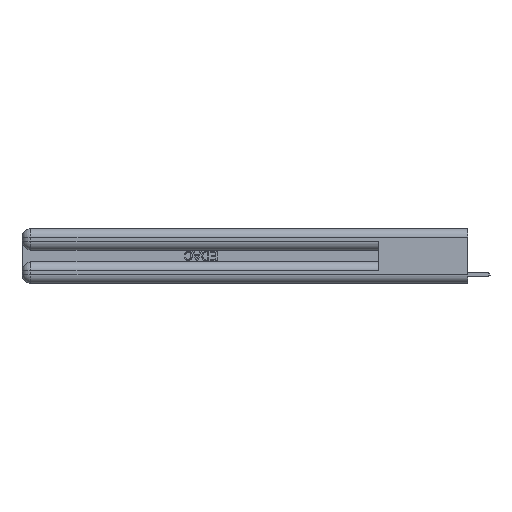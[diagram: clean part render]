
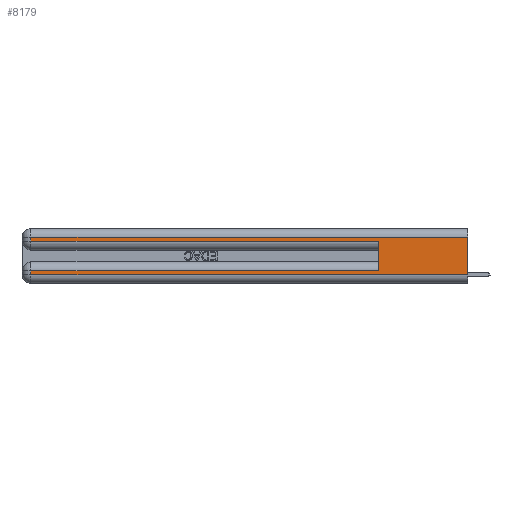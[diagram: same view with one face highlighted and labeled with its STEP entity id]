
A CAD part, left-side view. The second image highlights one B-rep face of the part: STEP entity #8179.
In plain terms, the highlighted planar face has unit normal (-1, 0, 0).
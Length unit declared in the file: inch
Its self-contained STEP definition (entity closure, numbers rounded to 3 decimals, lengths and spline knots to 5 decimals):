
#198 = CARTESIAN_POINT ( 'NONE',  ( 0., 0., 0.06 ) ) ;
#543 = CARTESIAN_POINT ( 'NONE',  ( 0., 2.94, 0.37 ) ) ;
#770 = CARTESIAN_POINT ( 'NONE',  ( 0., 0., 0.31 ) ) ;
#833 = VERTEX_POINT ( 'NONE', #26315 ) ;
#1070 = ORIENTED_EDGE ( 'NONE', *, *, #5201, .T. ) ;
#1204 = VECTOR ( 'NONE', #26337, 39.37008 ) ;
#1391 = VERTEX_POINT ( 'NONE', #16134 ) ;
#1666 = ORIENTED_EDGE ( 'NONE', *, *, #19985, .T. ) ;
#2874 = ORIENTED_EDGE ( 'NONE', *, *, #17030, .T. ) ;
#2978 = AXIS2_PLACEMENT_3D ( 'NONE', #25072, #17737, #20302 ) ;
#3149 = CARTESIAN_POINT ( 'NONE',  ( 0., 2.94, 0.31 ) ) ;
#3620 = PLANE ( 'NONE',  #2978 ) ;
#3633 = LINE ( 'NONE', #27394, #27458 ) ;
#4206 = ORIENTED_EDGE ( 'NONE', *, *, #17694, .F. ) ;
#4421 = VECTOR ( 'NONE', #28871, 39.37008 ) ;
#5201 = EDGE_CURVE ( 'NONE', #1391, #10972, #11929, .T. ) ;
#6618 = CARTESIAN_POINT ( 'NONE',  ( 0., 0., 0.285 ) ) ;
#6822 = VECTOR ( 'NONE', #21873, 39.37008 ) ;
#6922 = VECTOR ( 'NONE', #17334, 39.37008 ) ;
#7371 = CARTESIAN_POINT ( 'NONE',  ( 0., 2.94, 0.06 ) ) ;
#7586 = VERTEX_POINT ( 'NONE', #7646 ) ;
#7646 = CARTESIAN_POINT ( 'NONE',  ( 0., 0.6, 0.285 ) ) ;
#8179 = ADVANCED_FACE ( 'NONE', ( #18032 ), #3620, .F. ) ;
#8916 = LINE ( 'NONE', #24292, #22988 ) ;
#9814 = LINE ( 'NONE', #28670, #6922 ) ;
#9959 = EDGE_CURVE ( 'NONE', #13975, #1391, #9814, .T. ) ;
#10230 = LINE ( 'NONE', #770, #1204 ) ;
#10925 = LINE ( 'NONE', #6618, #19636 ) ;
#10972 = VERTEX_POINT ( 'NONE', #7371 ) ;
#11510 = CARTESIAN_POINT ( 'NONE',  ( 0., 2.94, 0.285 ) ) ;
#11929 = LINE ( 'NONE', #21104, #16793 ) ;
#12183 = VERTEX_POINT ( 'NONE', #18018 ) ;
#13900 = CARTESIAN_POINT ( 'NONE',  ( 0., 0.6, 0.085 ) ) ;
#13975 = VERTEX_POINT ( 'NONE', #13900 ) ;
#14807 = EDGE_CURVE ( 'NONE', #10972, #833, #29083, .T. ) ;
#15764 = ORIENTED_EDGE ( 'NONE', *, *, #18170, .F. ) ;
#15989 = DIRECTION ( 'NONE',  ( 0., 0., 1. ) ) ;
#16134 = CARTESIAN_POINT ( 'NONE',  ( 0., 2.94, 0.085 ) ) ;
#16192 = ORIENTED_EDGE ( 'NONE', *, *, #14807, .T. ) ;
#16793 = VECTOR ( 'NONE', #17137, 39.37008 ) ;
#17030 = EDGE_CURVE ( 'NONE', #24422, #19929, #19507, .T. ) ;
#17137 = DIRECTION ( 'NONE',  ( 0., 0., -1. ) ) ;
#17334 = DIRECTION ( 'NONE',  ( 0., 1., 0. ) ) ;
#17694 = EDGE_CURVE ( 'NONE', #12183, #833, #3633, .T. ) ;
#17737 = DIRECTION ( 'NONE',  ( 1., 0., 0. ) ) ;
#18018 = CARTESIAN_POINT ( 'NONE',  ( 0., 0., 0.31 ) ) ;
#18032 = FACE_OUTER_BOUND ( 'NONE', #22688, .T. ) ;
#18044 = DIRECTION ( 'NONE',  ( 0., 0., -1. ) ) ;
#18170 = EDGE_CURVE ( 'NONE', #13975, #7586, #8916, .T. ) ;
#19507 = LINE ( 'NONE', #543, #4421 ) ;
#19636 = VECTOR ( 'NONE', #30207, 39.37008 ) ;
#19929 = VERTEX_POINT ( 'NONE', #11510 ) ;
#19985 = EDGE_CURVE ( 'NONE', #19929, #7586, #10925, .T. ) ;
#20302 = DIRECTION ( 'NONE',  ( 0., 0., -1. ) ) ;
#21104 = CARTESIAN_POINT ( 'NONE',  ( 0., 2.94, 0.37 ) ) ;
#21404 = ORIENTED_EDGE ( 'NONE', *, *, #9959, .T. ) ;
#21873 = DIRECTION ( 'NONE',  ( 0., -1., 0. ) ) ;
#22688 = EDGE_LOOP ( 'NONE', ( #4206, #26595, #2874, #1666, #15764, #21404, #1070, #16192 ) ) ;
#22988 = VECTOR ( 'NONE', #15989, 39.37008 ) ;
#24292 = CARTESIAN_POINT ( 'NONE',  ( 0., 0.6, 0.145 ) ) ;
#24422 = VERTEX_POINT ( 'NONE', #3149 ) ;
#25072 = CARTESIAN_POINT ( 'NONE',  ( 0., 0., 0.37 ) ) ;
#26315 = CARTESIAN_POINT ( 'NONE',  ( 0., 0., 0.06 ) ) ;
#26337 = DIRECTION ( 'NONE',  ( 0., 1., 0. ) ) ;
#26595 = ORIENTED_EDGE ( 'NONE', *, *, #27722, .T. ) ;
#27394 = CARTESIAN_POINT ( 'NONE',  ( 0., 0., 0.37 ) ) ;
#27458 = VECTOR ( 'NONE', #18044, 39.37008 ) ;
#27722 = EDGE_CURVE ( 'NONE', #12183, #24422, #10230, .T. ) ;
#28670 = CARTESIAN_POINT ( 'NONE',  ( 0., 0., 0.085 ) ) ;
#28871 = DIRECTION ( 'NONE',  ( 0., 0., -1. ) ) ;
#29083 = LINE ( 'NONE', #198, #6822 ) ;
#30207 = DIRECTION ( 'NONE',  ( 0., -1., 0. ) ) ;
